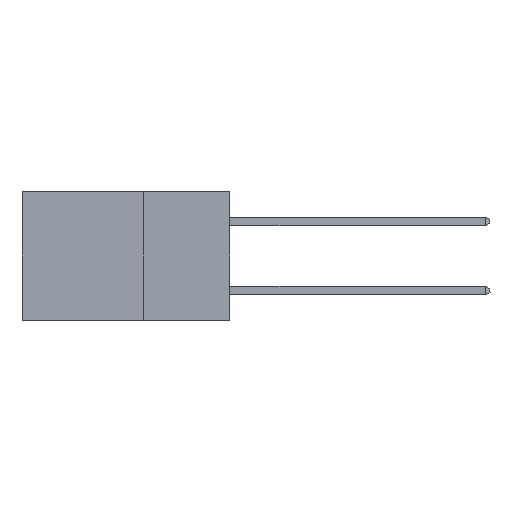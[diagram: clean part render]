
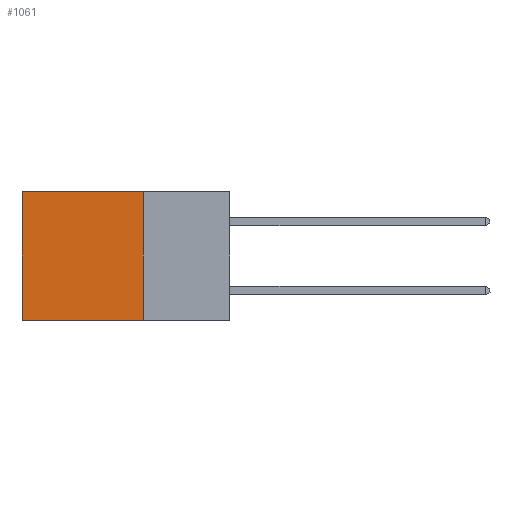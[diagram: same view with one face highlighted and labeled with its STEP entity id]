
A CAD part, left-side view. The second image highlights one B-rep face of the part: STEP entity #1061.
In plain terms, the highlighted planar face has unit normal (-1, 0, 0).
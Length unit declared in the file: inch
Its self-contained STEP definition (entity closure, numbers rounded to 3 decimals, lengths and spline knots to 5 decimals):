
#283 = DIRECTION ( 'NONE',  ( 0., 1., 0. ) ) ;
#703 = VECTOR ( 'NONE', #7310, 39.37008 ) ;
#985 = CARTESIAN_POINT ( 'NONE',  ( 0.298, 0.25, -0.37 ) ) ;
#1061 = ADVANCED_FACE ( 'NONE', ( #4438 ), #14778, .F. ) ;
#2044 = ORIENTED_EDGE ( 'NONE', *, *, #15996, .T. ) ;
#3154 = LINE ( 'NONE', #9029, #5550 ) ;
#4269 = VECTOR ( 'NONE', #6428, 39.37008 ) ;
#4438 = FACE_OUTER_BOUND ( 'NONE', #11655, .T. ) ;
#4679 = DIRECTION ( 'NONE',  ( 0., 0., -1. ) ) ;
#5550 = VECTOR ( 'NONE', #283, 39.37008 ) ;
#5691 = VECTOR ( 'NONE', #4679, 39.37008 ) ;
#6048 = CARTESIAN_POINT ( 'NONE',  ( 0.298, 0.6, 0. ) ) ;
#6154 = DIRECTION ( 'NONE',  ( 0., 0., -1. ) ) ;
#6320 = ORIENTED_EDGE ( 'NONE', *, *, #6357, .F. ) ;
#6357 = EDGE_CURVE ( 'NONE', #10535, #7486, #7602, .T. ) ;
#6428 = DIRECTION ( 'NONE',  ( 0., 0., -1. ) ) ;
#6586 = EDGE_CURVE ( 'NONE', #7486, #7473, #15265, .T. ) ;
#7310 = DIRECTION ( 'NONE',  ( 0., 1., 0. ) ) ;
#7473 = VERTEX_POINT ( 'NONE', #9920 ) ;
#7486 = VERTEX_POINT ( 'NONE', #10035 ) ;
#7602 = LINE ( 'NONE', #12739, #4269 ) ;
#7782 = CARTESIAN_POINT ( 'NONE',  ( 0.298, 0.25, 0. ) ) ;
#9029 = CARTESIAN_POINT ( 'NONE',  ( 0.298, 0.25, 0. ) ) ;
#9259 = ORIENTED_EDGE ( 'NONE', *, *, #6586, .F. ) ;
#9827 = DIRECTION ( 'NONE',  ( 1., 0., 0. ) ) ;
#9920 = CARTESIAN_POINT ( 'NONE',  ( 0.298, 0.6, -0.37 ) ) ;
#10035 = CARTESIAN_POINT ( 'NONE',  ( 0.298, 0.25, -0.37 ) ) ;
#10535 = VERTEX_POINT ( 'NONE', #7782 ) ;
#11655 = EDGE_LOOP ( 'NONE', ( #14022, #9259, #6320, #2044 ) ) ;
#11826 = LINE ( 'NONE', #6048, #5691 ) ;
#12739 = CARTESIAN_POINT ( 'NONE',  ( 0.298, 0.25, 0. ) ) ;
#12850 = VERTEX_POINT ( 'NONE', #15297 ) ;
#13718 = CARTESIAN_POINT ( 'NONE',  ( 0.298, 0.25, 0. ) ) ;
#13830 = AXIS2_PLACEMENT_3D ( 'NONE', #13718, #9827, #6154 ) ;
#14022 = ORIENTED_EDGE ( 'NONE', *, *, #15698, .T. ) ;
#14778 = PLANE ( 'NONE',  #13830 ) ;
#15265 = LINE ( 'NONE', #985, #703 ) ;
#15297 = CARTESIAN_POINT ( 'NONE',  ( 0.298, 0.6, 0. ) ) ;
#15698 = EDGE_CURVE ( 'NONE', #12850, #7473, #11826, .T. ) ;
#15996 = EDGE_CURVE ( 'NONE', #10535, #12850, #3154, .T. ) ;
